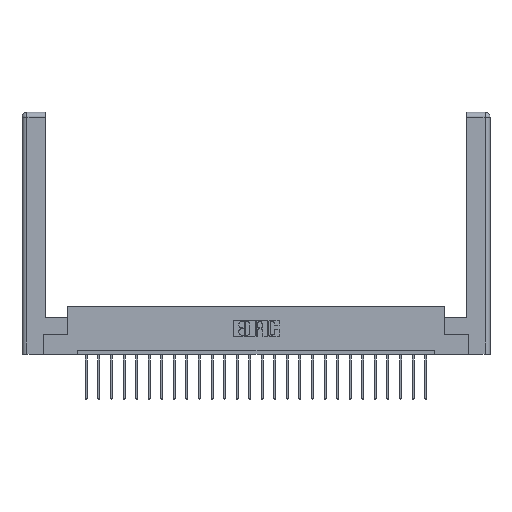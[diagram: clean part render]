
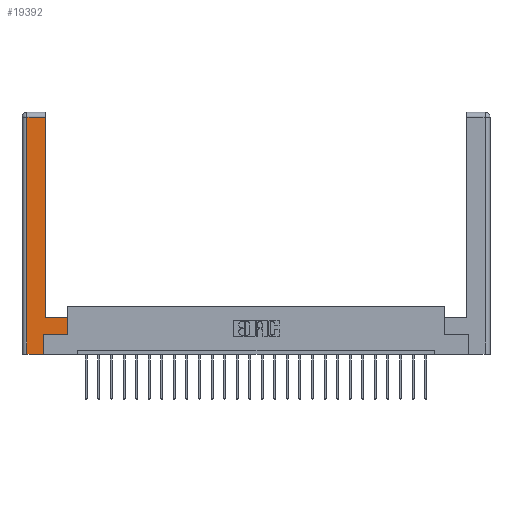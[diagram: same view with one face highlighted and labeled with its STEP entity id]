
A CAD part, top view. The second image highlights one B-rep face of the part: STEP entity #19392.
In plain terms, the highlighted planar face has unit normal (0, 0, 1).
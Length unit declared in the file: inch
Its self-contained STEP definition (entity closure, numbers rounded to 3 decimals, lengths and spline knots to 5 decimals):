
#119 = CARTESIAN_POINT ( 'NONE',  ( 0.565, 0.45, 0. ) ) ;
#160 = ORIENTED_EDGE ( 'NONE', *, *, #249, .T. ) ;
#201 = VECTOR ( 'NONE', #9056, 39.37008 ) ;
#249 = EDGE_CURVE ( 'NONE', #2718, #5330, #3043, .T. ) ;
#509 = ORIENTED_EDGE ( 'NONE', *, *, #8831, .T. ) ;
#838 = PLANE ( 'NONE',  #3478 ) ;
#1347 = EDGE_CURVE ( 'NONE', #4936, #12864, #19493, .T. ) ;
#1405 = DIRECTION ( 'NONE',  ( 0., 1., 0. ) ) ;
#1781 = VECTOR ( 'NONE', #5273, 39.37008 ) ;
#2126 = ORIENTED_EDGE ( 'NONE', *, *, #16153, .T. ) ;
#2718 = VERTEX_POINT ( 'NONE', #17015 ) ;
#3043 = LINE ( 'NONE', #22813, #14917 ) ;
#3196 = LINE ( 'NONE', #119, #19676 ) ;
#3478 = AXIS2_PLACEMENT_3D ( 'NONE', #24107, #4668, #24200 ) ;
#3896 = DIRECTION ( 'NONE',  ( 1., 0., 0. ) ) ;
#4668 = DIRECTION ( 'NONE',  ( 0., 0., -1. ) ) ;
#4922 = CARTESIAN_POINT ( 'NONE',  ( 0.295, 3., 0. ) ) ;
#4936 = VERTEX_POINT ( 'NONE', #7474 ) ;
#5273 = DIRECTION ( 'NONE',  ( 1., 0., 0. ) ) ;
#5330 = VERTEX_POINT ( 'NONE', #15188 ) ;
#5564 = EDGE_LOOP ( 'NONE', ( #23049, #160, #509, #23121, #8649, #2126, #6488, #24970 ) ) ;
#5968 = VECTOR ( 'NONE', #1405, 39.37008 ) ;
#6488 = ORIENTED_EDGE ( 'NONE', *, *, #11271, .T. ) ;
#6965 = CARTESIAN_POINT ( 'NONE',  ( 0.565, 0.245, 0. ) ) ;
#7471 = CARTESIAN_POINT ( 'NONE',  ( 0.565, 0.245, 0. ) ) ;
#7474 = CARTESIAN_POINT ( 'NONE',  ( 0.0615, 0., 0. ) ) ;
#7734 = CARTESIAN_POINT ( 'NONE',  ( 0.265, 0., 0. ) ) ;
#8647 = EDGE_CURVE ( 'NONE', #12864, #9518, #11160, .T. ) ;
#8649 = ORIENTED_EDGE ( 'NONE', *, *, #8647, .T. ) ;
#8831 = EDGE_CURVE ( 'NONE', #5330, #4936, #16330, .T. ) ;
#8850 = DIRECTION ( 'NONE',  ( 0., 1., 0. ) ) ;
#9056 = DIRECTION ( 'NONE',  ( -1., 0., 0. ) ) ;
#9445 = CARTESIAN_POINT ( 'NONE',  ( 0.265, 0.245, 0. ) ) ;
#9518 = VERTEX_POINT ( 'NONE', #9445 ) ;
#9556 = FACE_OUTER_BOUND ( 'NONE', #5564, .T. ) ;
#10999 = CARTESIAN_POINT ( 'NONE',  ( 0.265, 0., 0. ) ) ;
#11160 = LINE ( 'NONE', #14951, #5968 ) ;
#11271 = EDGE_CURVE ( 'NONE', #16210, #16062, #3196, .T. ) ;
#11376 = DIRECTION ( 'NONE',  ( -1., 0., 0. ) ) ;
#11636 = DIRECTION ( 'NONE',  ( 0., -1., 0. ) ) ;
#11639 = DIRECTION ( 'NONE',  ( 0., 1., 0. ) ) ;
#12306 = CARTESIAN_POINT ( 'NONE',  ( 0.295, 0.45, 0. ) ) ;
#12864 = VERTEX_POINT ( 'NONE', #10999 ) ;
#12907 = EDGE_CURVE ( 'NONE', #17121, #2718, #13794, .T. ) ;
#13151 = CARTESIAN_POINT ( 'NONE',  ( 0.295, 0.45, 0. ) ) ;
#13794 = LINE ( 'NONE', #4922, #23537 ) ;
#14840 = LINE ( 'NONE', #13151, #201 ) ;
#14917 = VECTOR ( 'NONE', #11376, 39.37008 ) ;
#14951 = CARTESIAN_POINT ( 'NONE',  ( 0.265, 0.245, 0. ) ) ;
#15130 = VECTOR ( 'NONE', #11636, 39.37008 ) ;
#15188 = CARTESIAN_POINT ( 'NONE',  ( 0.0615, 2.94, 0. ) ) ;
#16062 = VERTEX_POINT ( 'NONE', #16862 ) ;
#16153 = EDGE_CURVE ( 'NONE', #9518, #16210, #23138, .T. ) ;
#16210 = VERTEX_POINT ( 'NONE', #7471 ) ;
#16330 = LINE ( 'NONE', #25030, #15130 ) ;
#16862 = CARTESIAN_POINT ( 'NONE',  ( 0.565, 0.45, 0. ) ) ;
#17015 = CARTESIAN_POINT ( 'NONE',  ( 0.295, 2.94, 0. ) ) ;
#17121 = VERTEX_POINT ( 'NONE', #12306 ) ;
#19392 = ADVANCED_FACE ( 'NONE', ( #9556 ), #838, .F. ) ;
#19493 = LINE ( 'NONE', #7734, #23145 ) ;
#19676 = VECTOR ( 'NONE', #11639, 39.37008 ) ;
#22813 = CARTESIAN_POINT ( 'NONE',  ( 0.0615, 2.94, 0. ) ) ;
#23049 = ORIENTED_EDGE ( 'NONE', *, *, #12907, .T. ) ;
#23121 = ORIENTED_EDGE ( 'NONE', *, *, #1347, .T. ) ;
#23138 = LINE ( 'NONE', #6965, #1781 ) ;
#23145 = VECTOR ( 'NONE', #3896, 39.37008 ) ;
#23537 = VECTOR ( 'NONE', #8850, 39.37008 ) ;
#24107 = CARTESIAN_POINT ( 'NONE',  ( 0., 0., 0. ) ) ;
#24200 = DIRECTION ( 'NONE',  ( -1., 0., 0. ) ) ;
#24970 = ORIENTED_EDGE ( 'NONE', *, *, #24990, .T. ) ;
#24990 = EDGE_CURVE ( 'NONE', #16062, #17121, #14840, .T. ) ;
#25030 = CARTESIAN_POINT ( 'NONE',  ( 0.0615, 0., 0. ) ) ;
